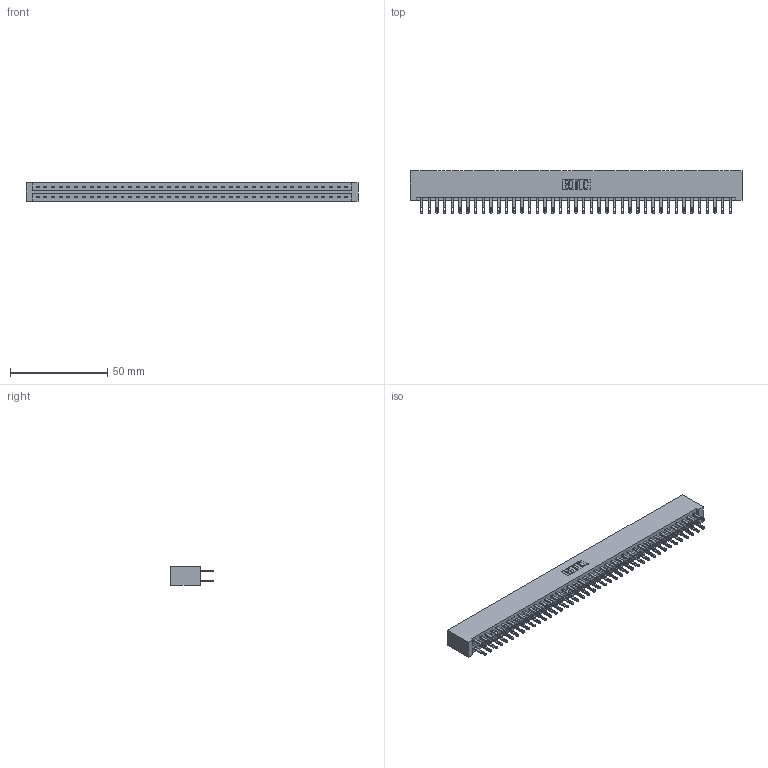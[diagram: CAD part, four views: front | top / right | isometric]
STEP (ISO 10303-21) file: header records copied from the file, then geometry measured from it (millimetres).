
FILE_DESCRIPTION (( 'STEP AP203' ), '1' );
FILE_NAME ('337-082-500-201.STEP', '2019-10-10T12:41:32', ( '' ), ( '' ), 'SwSTEP 2.0', 'SolidWorks 2016', '' );
FILE_SCHEMA (( 'CONFIG_CONTROL_DESIGN' ));
Length unit declared in the file: inch
Products named in the file (3): 337 Part_No Mounting Lugs; 345-292-001_345-293-100; 337-082-500-201
Assembly tree (83 placements, depth 2):
  337-082-500-201
    337 Part_No Mounting Lugs
    345-292-001_345-293-100  x82
Bounding box: 170.33 x 21.85 x 9.4 mm (x, y, z)
Volume: 18949 mm3; surface area: 22378.1 mm2
Topology: 83 solids, 83 shells, 4206 faces, 12833 edges, 8554 vertices
Faces by surface type: plane 2690, cylinder 1516
Entity records: 31571 total; most frequent: CARTESIAN_POINT 5318, ORIENTED_EDGE 5254, DIRECTION 4519, EDGE_CURVE 2627, LINE 2503, VECTOR 2503, VERTEX_POINT 1750, AXIS2_PLACEMENT_3D 1008
